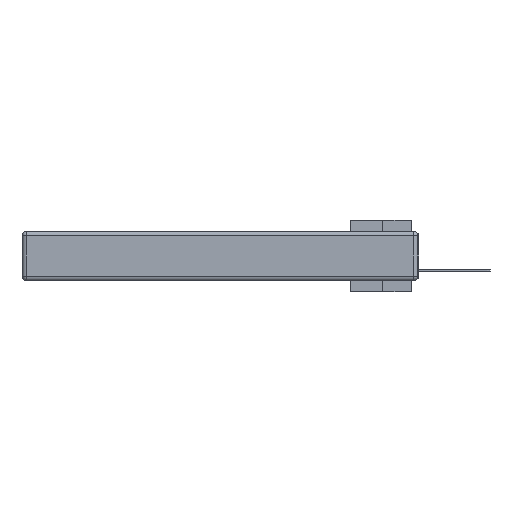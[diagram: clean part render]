
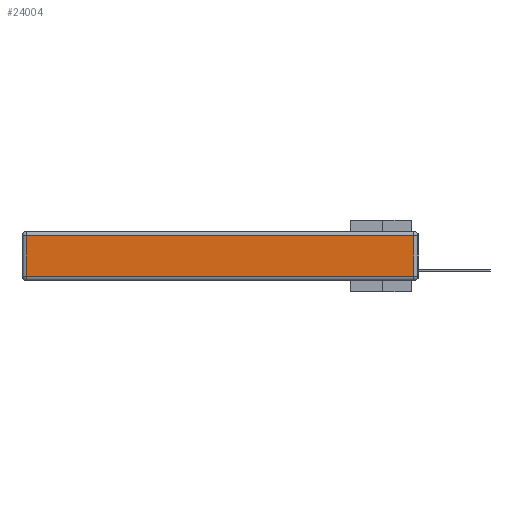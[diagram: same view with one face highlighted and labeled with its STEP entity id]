
A CAD part, left-side view. The second image highlights one B-rep face of the part: STEP entity #24004.
In plain terms, the highlighted planar face has unit normal (-1, 0, 0).
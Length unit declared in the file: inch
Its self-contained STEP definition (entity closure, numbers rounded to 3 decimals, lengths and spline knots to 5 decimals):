
#1518 = DIRECTION ( 'NONE',  ( 0., -1., 0. ) ) ;
#2677 = EDGE_CURVE ( 'NONE', #6448, #18749, #3562, .T. ) ;
#2699 = ORIENTED_EDGE ( 'NONE', *, *, #2677, .T. ) ;
#2870 = ORIENTED_EDGE ( 'NONE', *, *, #5316, .T. ) ;
#3562 = LINE ( 'NONE', #10773, #13502 ) ;
#3708 = CARTESIAN_POINT ( 'NONE',  ( 0., 0.03, -0.03 ) ) ;
#4375 = EDGE_CURVE ( 'NONE', #18749, #23999, #21808, .T. ) ;
#5316 = EDGE_CURVE ( 'NONE', #23999, #26695, #23483, .T. ) ;
#5465 = DIRECTION ( 'NONE',  ( 0., 0., 1. ) ) ;
#5684 = EDGE_CURVE ( 'NONE', #26695, #6448, #29040, .T. ) ;
#5893 = VECTOR ( 'NONE', #19622, 39.37008 ) ;
#6448 = VERTEX_POINT ( 'NONE', #3708 ) ;
#7167 = CARTESIAN_POINT ( 'NONE',  ( 0., 0., -0.343 ) ) ;
#10773 = CARTESIAN_POINT ( 'NONE',  ( 0., 2.75, -0.03 ) ) ;
#10940 = ORIENTED_EDGE ( 'NONE', *, *, #4375, .T. ) ;
#11382 = CARTESIAN_POINT ( 'NONE',  ( 0., 2.72, -0.03 ) ) ;
#13502 = VECTOR ( 'NONE', #17689, 39.37008 ) ;
#15880 = DIRECTION ( 'NONE',  ( 0., 0., 1. ) ) ;
#17336 = CARTESIAN_POINT ( 'NONE',  ( 0., 0., -0.313 ) ) ;
#17568 = CARTESIAN_POINT ( 'NONE',  ( 0., 0.03, -0.313 ) ) ;
#17689 = DIRECTION ( 'NONE',  ( 0., 1., 0. ) ) ;
#18163 = PLANE ( 'NONE',  #25429 ) ;
#18749 = VERTEX_POINT ( 'NONE', #11382 ) ;
#18941 = VECTOR ( 'NONE', #1518, 39.37008 ) ;
#19622 = DIRECTION ( 'NONE',  ( 0., 0., -1. ) ) ;
#20914 = FACE_OUTER_BOUND ( 'NONE', #28820, .T. ) ;
#21808 = LINE ( 'NONE', #21955, #5893 ) ;
#21955 = CARTESIAN_POINT ( 'NONE',  ( 0., 2.72, -0.343 ) ) ;
#22848 = CARTESIAN_POINT ( 'NONE',  ( 0., 2.72, -0.313 ) ) ;
#22949 = DIRECTION ( 'NONE',  ( -1., 0., 0. ) ) ;
#23483 = LINE ( 'NONE', #17336, #18941 ) ;
#23897 = ORIENTED_EDGE ( 'NONE', *, *, #5684, .T. ) ;
#23999 = VERTEX_POINT ( 'NONE', #22848 ) ;
#24004 = ADVANCED_FACE ( 'NONE', ( #20914 ), #18163, .T. ) ;
#25148 = VECTOR ( 'NONE', #15880, 39.37008 ) ;
#25429 = AXIS2_PLACEMENT_3D ( 'NONE', #7167, #22949, #5465 ) ;
#26695 = VERTEX_POINT ( 'NONE', #17568 ) ;
#26811 = CARTESIAN_POINT ( 'NONE',  ( 0., 0.03, -0.343 ) ) ;
#28820 = EDGE_LOOP ( 'NONE', ( #2870, #23897, #2699, #10940 ) ) ;
#29040 = LINE ( 'NONE', #26811, #25148 ) ;
